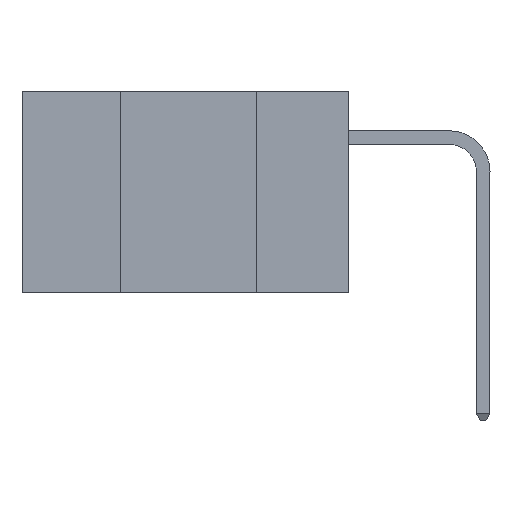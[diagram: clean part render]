
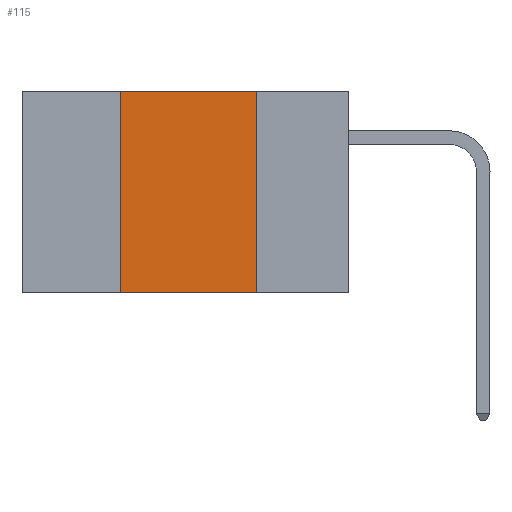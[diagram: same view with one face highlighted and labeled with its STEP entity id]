
A CAD part, left-side view. The second image highlights one B-rep face of the part: STEP entity #115.
In plain terms, the highlighted planar face has unit normal (-1, 0, 0).
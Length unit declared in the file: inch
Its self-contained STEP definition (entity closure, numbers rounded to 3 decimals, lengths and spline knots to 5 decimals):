
#34 = ORIENTED_EDGE ( 'NONE', *, *, #4940, .F. ) ;
#115 = ADVANCED_FACE ( 'NONE', ( #9196 ), #5251, .F. ) ;
#209 = CARTESIAN_POINT ( 'NONE',  ( 0., 0.17, -0.37 ) ) ;
#259 = VECTOR ( 'NONE', #4453, 39.37008 ) ;
#444 = VERTEX_POINT ( 'NONE', #10326 ) ;
#563 = LINE ( 'NONE', #8504, #259 ) ;
#646 = VECTOR ( 'NONE', #5515, 39.37008 ) ;
#783 = LINE ( 'NONE', #4658, #646 ) ;
#1253 = ORIENTED_EDGE ( 'NONE', *, *, #8967, .F. ) ;
#1417 = ORIENTED_EDGE ( 'NONE', *, *, #2591, .F. ) ;
#1514 = CARTESIAN_POINT ( 'NONE',  ( 0., 0.42, -0.37 ) ) ;
#2003 = ORIENTED_EDGE ( 'NONE', *, *, #8588, .T. ) ;
#2591 = EDGE_CURVE ( 'NONE', #6806, #9634, #4732, .T. ) ;
#2724 = DIRECTION ( 'NONE',  ( 1., 0., 0. ) ) ;
#2878 = DIRECTION ( 'NONE',  ( 0., 0., -1. ) ) ;
#3499 = DIRECTION ( 'NONE',  ( 0., 0., 1. ) ) ;
#3684 = CARTESIAN_POINT ( 'NONE',  ( 0., 0.42, 0. ) ) ;
#4290 = EDGE_LOOP ( 'NONE', ( #34, #1253, #1417, #2003 ) ) ;
#4453 = DIRECTION ( 'NONE',  ( 0., -1., 0. ) ) ;
#4501 = CARTESIAN_POINT ( 'NONE',  ( 0., 0.17, 0. ) ) ;
#4593 = VECTOR ( 'NONE', #3499, 39.37008 ) ;
#4658 = CARTESIAN_POINT ( 'NONE',  ( 0., 0.6, -0.37 ) ) ;
#4732 = LINE ( 'NONE', #9906, #4593 ) ;
#4940 = EDGE_CURVE ( 'NONE', #444, #6689, #8335, .T. ) ;
#5251 = PLANE ( 'NONE',  #6316 ) ;
#5515 = DIRECTION ( 'NONE',  ( 0., -1., 0. ) ) ;
#6316 = AXIS2_PLACEMENT_3D ( 'NONE', #10350, #2724, #2878 ) ;
#6689 = VERTEX_POINT ( 'NONE', #209 ) ;
#6806 = VERTEX_POINT ( 'NONE', #1514 ) ;
#8305 = VECTOR ( 'NONE', #9305, 39.37008 ) ;
#8335 = LINE ( 'NONE', #4501, #8305 ) ;
#8504 = CARTESIAN_POINT ( 'NONE',  ( 0., 0.6, 0. ) ) ;
#8588 = EDGE_CURVE ( 'NONE', #6806, #6689, #783, .T. ) ;
#8967 = EDGE_CURVE ( 'NONE', #9634, #444, #563, .T. ) ;
#9196 = FACE_OUTER_BOUND ( 'NONE', #4290, .T. ) ;
#9305 = DIRECTION ( 'NONE',  ( 0., 0., -1. ) ) ;
#9634 = VERTEX_POINT ( 'NONE', #3684 ) ;
#9906 = CARTESIAN_POINT ( 'NONE',  ( 0., 0.42, 0. ) ) ;
#10326 = CARTESIAN_POINT ( 'NONE',  ( 0., 0.17, 0. ) ) ;
#10350 = CARTESIAN_POINT ( 'NONE',  ( 0., 0.6, 0. ) ) ;
